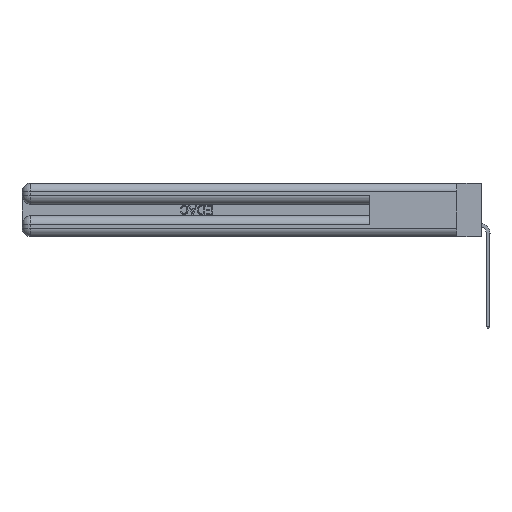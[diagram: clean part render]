
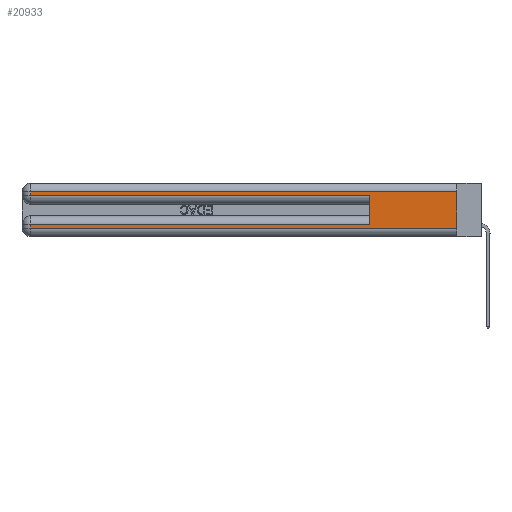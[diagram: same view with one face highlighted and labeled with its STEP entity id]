
A CAD part, left-side view. The second image highlights one B-rep face of the part: STEP entity #20933.
In plain terms, the highlighted planar face has unit normal (-1, 0, 0).
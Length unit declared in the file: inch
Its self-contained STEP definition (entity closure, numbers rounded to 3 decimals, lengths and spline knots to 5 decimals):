
#97 = DIRECTION ( 'NONE',  ( 0., 0., -1. ) ) ;
#285 = LINE ( 'NONE', #17223, #25482 ) ;
#394 = CARTESIAN_POINT ( 'NONE',  ( 0., 2.94, 0.37 ) ) ;
#1020 = EDGE_CURVE ( 'NONE', #4657, #42232, #27518, .T. ) ;
#2357 = VERTEX_POINT ( 'NONE', #3754 ) ;
#3088 = FACE_OUTER_BOUND ( 'NONE', #28739, .T. ) ;
#3499 = CARTESIAN_POINT ( 'NONE',  ( 0., 0., 0.285 ) ) ;
#3754 = CARTESIAN_POINT ( 'NONE',  ( 0., 2.94, 0.085 ) ) ;
#4008 = CARTESIAN_POINT ( 'NONE',  ( 0., 0.6, 0.085 ) ) ;
#4183 = DIRECTION ( 'NONE',  ( 0., 1., 0. ) ) ;
#4657 = VERTEX_POINT ( 'NONE', #28906 ) ;
#5715 = CARTESIAN_POINT ( 'NONE',  ( 0., 0., 0.06 ) ) ;
#6127 = DIRECTION ( 'NONE',  ( 0., -1., 0. ) ) ;
#6477 = EDGE_CURVE ( 'NONE', #42232, #40123, #32234, .T. ) ;
#6496 = LINE ( 'NONE', #10157, #20851 ) ;
#7208 = LINE ( 'NONE', #11113, #14352 ) ;
#8330 = CARTESIAN_POINT ( 'NONE',  ( 0., 0., 0.31 ) ) ;
#8628 = LINE ( 'NONE', #20528, #10652 ) ;
#10157 = CARTESIAN_POINT ( 'NONE',  ( 0., 0., 0.37 ) ) ;
#10652 = VECTOR ( 'NONE', #17357, 39.37008 ) ;
#11113 = CARTESIAN_POINT ( 'NONE',  ( 0., 0.6, 0.145 ) ) ;
#11662 = VECTOR ( 'NONE', #6127, 39.37008 ) ;
#12697 = CARTESIAN_POINT ( 'NONE',  ( 0., 0.6, 0.285 ) ) ;
#13258 = EDGE_CURVE ( 'NONE', #16535, #40123, #7208, .T. ) ;
#13996 = DIRECTION ( 'NONE',  ( 0., 0., -1. ) ) ;
#14352 = VECTOR ( 'NONE', #20747, 39.37008 ) ;
#15240 = CARTESIAN_POINT ( 'NONE',  ( 0., 2.94, 0.06 ) ) ;
#15654 = EDGE_CURVE ( 'NONE', #27192, #18003, #8628, .T. ) ;
#16079 = CARTESIAN_POINT ( 'NONE',  ( 0., 2.94, 0.37 ) ) ;
#16392 = CARTESIAN_POINT ( 'NONE',  ( 0., 0., 0.31 ) ) ;
#16535 = VERTEX_POINT ( 'NONE', #4008 ) ;
#16757 = EDGE_CURVE ( 'NONE', #32882, #18003, #6496, .T. ) ;
#17001 = ORIENTED_EDGE ( 'NONE', *, *, #13258, .F. ) ;
#17223 = CARTESIAN_POINT ( 'NONE',  ( 0., 0., 0.085 ) ) ;
#17357 = DIRECTION ( 'NONE',  ( 0., -1., 0. ) ) ;
#18003 = VERTEX_POINT ( 'NONE', #5715 ) ;
#18904 = ORIENTED_EDGE ( 'NONE', *, *, #21171, .T. ) ;
#19524 = EDGE_CURVE ( 'NONE', #2357, #27192, #29907, .T. ) ;
#19531 = DIRECTION ( 'NONE',  ( 0., 0., -1. ) ) ;
#20528 = CARTESIAN_POINT ( 'NONE',  ( 0., 0., 0.06 ) ) ;
#20529 = LINE ( 'NONE', #8330, #28205 ) ;
#20747 = DIRECTION ( 'NONE',  ( 0., 0., 1. ) ) ;
#20851 = VECTOR ( 'NONE', #19531, 39.37008 ) ;
#20933 = ADVANCED_FACE ( 'NONE', ( #3088 ), #26813, .F. ) ;
#21171 = EDGE_CURVE ( 'NONE', #32882, #4657, #20529, .T. ) ;
#21197 = VECTOR ( 'NONE', #13996, 39.37008 ) ;
#23223 = ORIENTED_EDGE ( 'NONE', *, *, #6477, .T. ) ;
#23352 = CARTESIAN_POINT ( 'NONE',  ( 0., 0., 0.37 ) ) ;
#24585 = ORIENTED_EDGE ( 'NONE', *, *, #1020, .T. ) ;
#25482 = VECTOR ( 'NONE', #4183, 39.37008 ) ;
#26143 = ORIENTED_EDGE ( 'NONE', *, *, #16757, .F. ) ;
#26158 = DIRECTION ( 'NONE',  ( 0., 0., -1. ) ) ;
#26813 = PLANE ( 'NONE',  #31300 ) ;
#27192 = VERTEX_POINT ( 'NONE', #15240 ) ;
#27518 = LINE ( 'NONE', #16079, #38842 ) ;
#27521 = ORIENTED_EDGE ( 'NONE', *, *, #15654, .T. ) ;
#28205 = VECTOR ( 'NONE', #34114, 39.37008 ) ;
#28739 = EDGE_LOOP ( 'NONE', ( #26143, #18904, #24585, #23223, #17001, #29721, #34624, #27521 ) ) ;
#28906 = CARTESIAN_POINT ( 'NONE',  ( 0., 2.94, 0.31 ) ) ;
#29146 = CARTESIAN_POINT ( 'NONE',  ( 0., 2.94, 0.285 ) ) ;
#29402 = EDGE_CURVE ( 'NONE', #16535, #2357, #285, .T. ) ;
#29721 = ORIENTED_EDGE ( 'NONE', *, *, #29402, .T. ) ;
#29907 = LINE ( 'NONE', #394, #21197 ) ;
#31300 = AXIS2_PLACEMENT_3D ( 'NONE', #23352, #37808, #97 ) ;
#32234 = LINE ( 'NONE', #3499, #11662 ) ;
#32882 = VERTEX_POINT ( 'NONE', #16392 ) ;
#34114 = DIRECTION ( 'NONE',  ( 0., 1., 0. ) ) ;
#34624 = ORIENTED_EDGE ( 'NONE', *, *, #19524, .T. ) ;
#37808 = DIRECTION ( 'NONE',  ( 1., 0., 0. ) ) ;
#38842 = VECTOR ( 'NONE', #26158, 39.37008 ) ;
#40123 = VERTEX_POINT ( 'NONE', #12697 ) ;
#42232 = VERTEX_POINT ( 'NONE', #29146 ) ;
